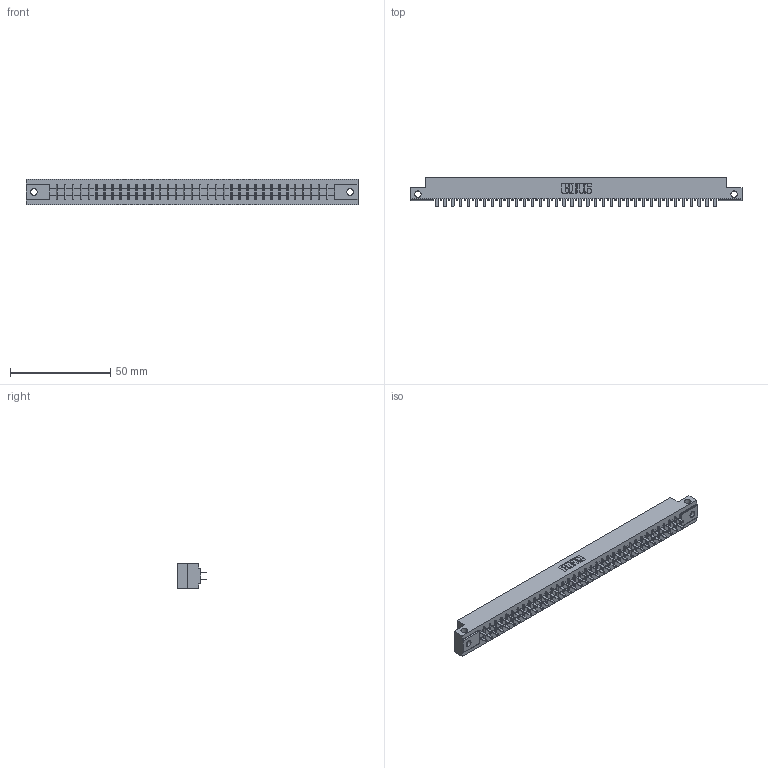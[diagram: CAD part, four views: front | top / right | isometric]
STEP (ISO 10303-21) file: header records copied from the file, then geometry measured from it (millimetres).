
FILE_DESCRIPTION (( 'STEP AP203' ), '1' );
FILE_NAME ('355-072-521-512.STEP', '2020-09-20T09:45:19', ( '' ), ( '' ), 'SwSTEP 2.0', 'SolidWorks 2020', '' );
FILE_SCHEMA (( 'CONFIG_CONTROL_DESIGN' ));
Length unit declared in the file: inch
Products named in the file (3): 305-290-001_521; 355-072-521-512; 305 Part_.128 Dia
Assembly tree (73 placements, depth 2):
  355-072-521-512
    305 Part_.128 Dia
    305-290-001_521  x72
Bounding box: 165.66 x 14.86 x 12.7 mm (x, y, z)
Volume: 16479.7 mm3; surface area: 21364.8 mm2
Topology: 73 solids, 73 shells, 3440 faces, 9820 edges, 6348 vertices
Faces by surface type: plane 2012, cylinder 1284, sphere 144
Entity records: 39995 total; most frequent: CARTESIAN_POINT 6666, ORIENTED_EDGE 6572, DIRECTION 6392, EDGE_CURVE 3286, LINE 2636, VECTOR 2636, VERTEX_POINT 2088, AXIS2_PLACEMENT_3D 1878
